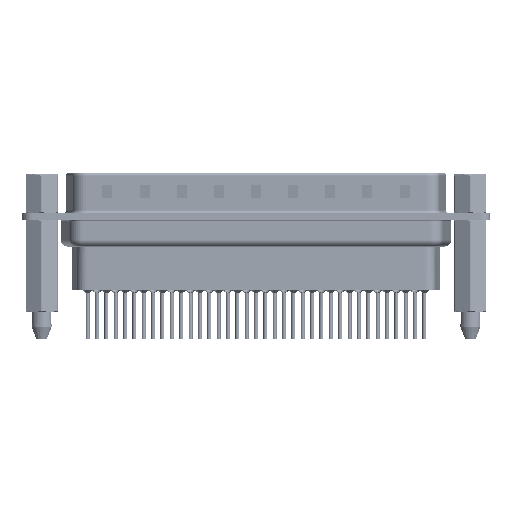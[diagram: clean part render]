
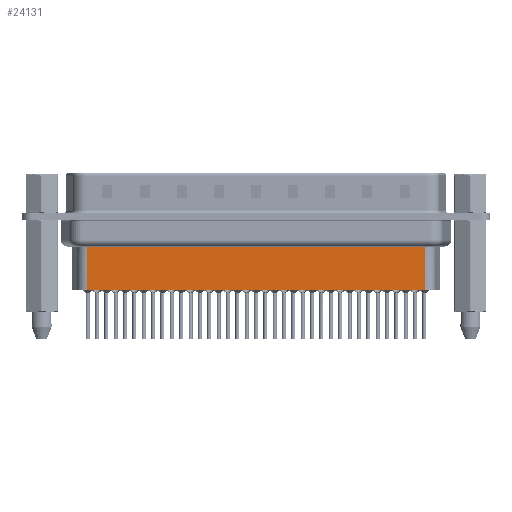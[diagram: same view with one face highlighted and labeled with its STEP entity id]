
A CAD part, front view. The second image highlights one B-rep face of the part: STEP entity #24131.
In plain terms, the highlighted planar face has unit normal (0, -1, 0).
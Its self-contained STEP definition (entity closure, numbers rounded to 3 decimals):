
#490 = DIRECTION ( 'NONE',  ( 1., 0., 0. ) ) ;
#1000 = LINE ( 'NONE', #17653, #30428 ) ;
#1298 = CARTESIAN_POINT ( 'NONE',  ( 56.794, -3.5, -3.1 ) ) ;
#1913 = VECTOR ( 'NONE', #33005, 1000. ) ;
#2396 = ORIENTED_EDGE ( 'NONE', *, *, #30036, .F. ) ;
#2937 = AXIS2_PLACEMENT_3D ( 'NONE', #26092, #23469, #490 ) ;
#3363 = EDGE_CURVE ( 'NONE', #36637, #17368, #5938, .T. ) ;
#4528 = ORIENTED_EDGE ( 'NONE', *, *, #3363, .T. ) ;
#5158 = CARTESIAN_POINT ( 'NONE',  ( 6.706, -3.5, -4.097 ) ) ;
#5938 = LINE ( 'NONE', #11187, #14353 ) ;
#9308 = VERTEX_POINT ( 'NONE', #35847 ) ;
#9743 = VECTOR ( 'NONE', #21840, 1000. ) ;
#11187 = CARTESIAN_POINT ( 'NONE',  ( 6.706, -3.5, -3.1 ) ) ;
#11213 = CARTESIAN_POINT ( 'NONE',  ( 56.794, -3.5, -4.097 ) ) ;
#11274 = CARTESIAN_POINT ( 'NONE',  ( 6.706, -3.5, -10.95 ) ) ;
#14353 = VECTOR ( 'NONE', #31182, 1000. ) ;
#14612 = VERTEX_POINT ( 'NONE', #11213 ) ;
#15078 = ORIENTED_EDGE ( 'NONE', *, *, #16880, .F. ) ;
#16880 = EDGE_CURVE ( 'NONE', #9308, #17368, #33362, .T. ) ;
#17368 = VERTEX_POINT ( 'NONE', #11274 ) ;
#17653 = CARTESIAN_POINT ( 'NONE',  ( 6.459, -3.5, -4.097 ) ) ;
#18668 = LINE ( 'NONE', #1298, #9743 ) ;
#21840 = DIRECTION ( 'NONE',  ( 0., 0., -1. ) ) ;
#22039 = EDGE_LOOP ( 'NONE', ( #2396, #25485, #4528, #15078 ) ) ;
#22149 = CARTESIAN_POINT ( 'NONE',  ( 6.706, -3.5, -10.95 ) ) ;
#23469 = DIRECTION ( 'NONE',  ( 0., -1., 0. ) ) ;
#24131 = ADVANCED_FACE ( 'NONE', ( #29090 ), #29267, .T. ) ;
#24638 = EDGE_CURVE ( 'NONE', #14612, #36637, #1000, .T. ) ;
#25485 = ORIENTED_EDGE ( 'NONE', *, *, #24638, .T. ) ;
#26092 = CARTESIAN_POINT ( 'NONE',  ( 6.706, -3.5, -3.1 ) ) ;
#28863 = DIRECTION ( 'NONE',  ( -1., 0., 0. ) ) ;
#29090 = FACE_OUTER_BOUND ( 'NONE', #22039, .T. ) ;
#29267 = PLANE ( 'NONE',  #2937 ) ;
#30036 = EDGE_CURVE ( 'NONE', #14612, #9308, #18668, .T. ) ;
#30428 = VECTOR ( 'NONE', #28863, 1000. ) ;
#31182 = DIRECTION ( 'NONE',  ( 0., 0., -1. ) ) ;
#33005 = DIRECTION ( 'NONE',  ( -1., 0., 0. ) ) ;
#33362 = LINE ( 'NONE', #22149, #1913 ) ;
#35847 = CARTESIAN_POINT ( 'NONE',  ( 56.794, -3.5, -10.95 ) ) ;
#36637 = VERTEX_POINT ( 'NONE', #5158 ) ;
